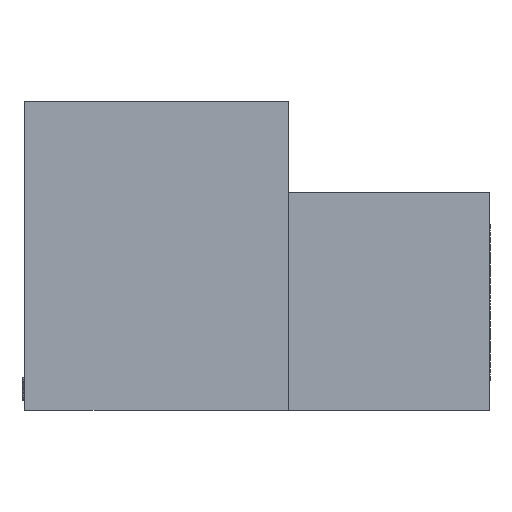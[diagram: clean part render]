
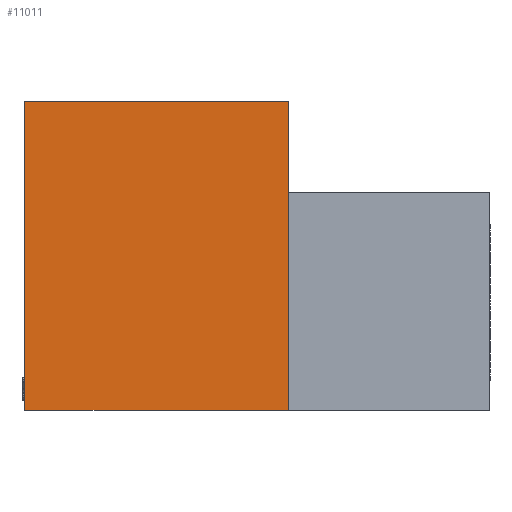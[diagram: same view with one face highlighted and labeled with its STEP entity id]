
A CAD part, left-side view. The second image highlights one B-rep face of the part: STEP entity #11011.
In plain terms, the highlighted planar face has unit normal (-1, 0, 0).
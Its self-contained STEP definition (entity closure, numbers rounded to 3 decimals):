
#887 = VERTEX_POINT ( 'NONE', #19675 ) ;
#3094 = CARTESIAN_POINT ( 'NONE',  ( 0., 0., 0. ) ) ;
#4318 = CARTESIAN_POINT ( 'NONE',  ( 0., 0., -13.487 ) ) ;
#5544 = FACE_OUTER_BOUND ( 'NONE', #38498, .T. ) ;
#9109 = CARTESIAN_POINT ( 'NONE',  ( 0., 0., 0. ) ) ;
#10048 = CARTESIAN_POINT ( 'NONE',  ( 0., -8.814, -13.487 ) ) ;
#10325 = DIRECTION ( 'NONE',  ( 0., 1., 0. ) ) ;
#10689 = LINE ( 'NONE', #3094, #20229 ) ;
#10896 = ORIENTED_EDGE ( 'NONE', *, *, #24702, .F. ) ;
#11011 = ADVANCED_FACE ( 'NONE', ( #5544 ), #34887, .F. ) ;
#13361 = LINE ( 'NONE', #21995, #40093 ) ;
#14424 = VERTEX_POINT ( 'NONE', #34335 ) ;
#15621 = DIRECTION ( 'NONE',  ( 0., -1., 0. ) ) ;
#15712 = LINE ( 'NONE', #10048, #33928 ) ;
#16373 = ORIENTED_EDGE ( 'NONE', *, *, #33439, .F. ) ;
#17799 = EDGE_CURVE ( 'NONE', #887, #14424, #41199, .T. ) ;
#19675 = CARTESIAN_POINT ( 'NONE',  ( 0., 11.506, -13.487 ) ) ;
#20229 = VECTOR ( 'NONE', #22647, 1000. ) ;
#20659 = ORIENTED_EDGE ( 'NONE', *, *, #26556, .F. ) ;
#21709 = VERTEX_POINT ( 'NONE', #4318 ) ;
#21995 = CARTESIAN_POINT ( 'NONE',  ( 0., 11.506, 0. ) ) ;
#22647 = DIRECTION ( 'NONE',  ( 0., 0., -1. ) ) ;
#24641 = DIRECTION ( 'NONE',  ( 0., 0., -1. ) ) ;
#24702 = EDGE_CURVE ( 'NONE', #14424, #28112, #13361, .T. ) ;
#26556 = EDGE_CURVE ( 'NONE', #28112, #21709, #10689, .T. ) ;
#26988 = CARTESIAN_POINT ( 'NONE',  ( 0., 11.506, -13.487 ) ) ;
#27139 = DIRECTION ( 'NONE',  ( 0., 0., 1. ) ) ;
#28112 = VERTEX_POINT ( 'NONE', #39424 ) ;
#33120 = AXIS2_PLACEMENT_3D ( 'NONE', #9109, #40840, #24641 ) ;
#33439 = EDGE_CURVE ( 'NONE', #21709, #887, #15712, .T. ) ;
#33928 = VECTOR ( 'NONE', #10325, 1000. ) ;
#34335 = CARTESIAN_POINT ( 'NONE',  ( 0., 11.506, 0. ) ) ;
#34887 = PLANE ( 'NONE',  #33120 ) ;
#38498 = EDGE_LOOP ( 'NONE', ( #16373, #20659, #10896, #40260 ) ) ;
#39424 = CARTESIAN_POINT ( 'NONE',  ( 0., 0., 0. ) ) ;
#40093 = VECTOR ( 'NONE', #15621, 1000. ) ;
#40260 = ORIENTED_EDGE ( 'NONE', *, *, #17799, .F. ) ;
#40840 = DIRECTION ( 'NONE',  ( 1., 0., 0. ) ) ;
#41199 = LINE ( 'NONE', #26988, #41684 ) ;
#41684 = VECTOR ( 'NONE', #27139, 1000. ) ;
